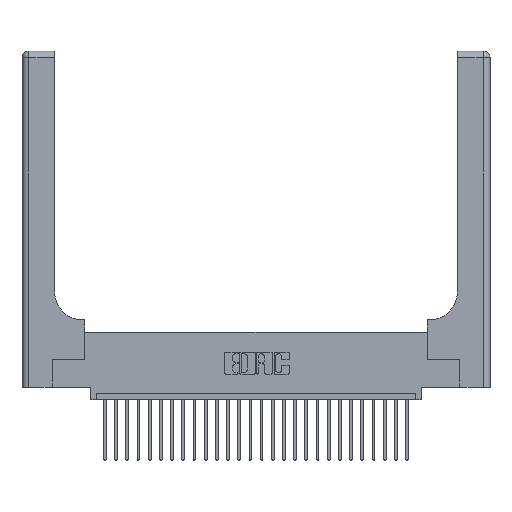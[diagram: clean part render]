
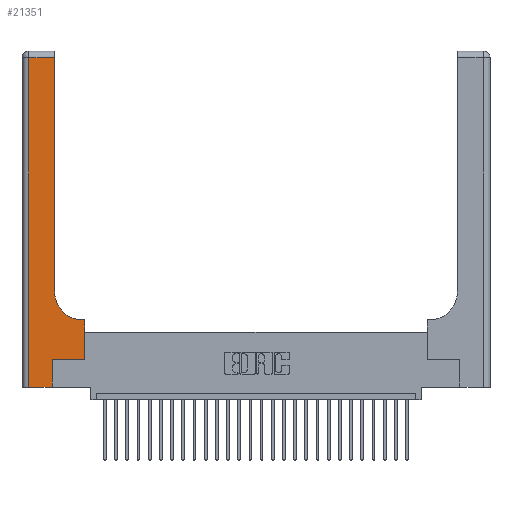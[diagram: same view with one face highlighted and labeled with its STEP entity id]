
A CAD part, top view. The second image highlights one B-rep face of the part: STEP entity #21351.
In plain terms, the highlighted planar face has unit normal (0, 0, 1).
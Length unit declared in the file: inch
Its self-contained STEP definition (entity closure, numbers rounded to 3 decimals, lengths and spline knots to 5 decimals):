
#375 = ORIENTED_EDGE ( 'NONE', *, *, #5644, .T. ) ;
#582 = CARTESIAN_POINT ( 'NONE',  ( 0.5585, 0.6, 0.37 ) ) ;
#1307 = VECTOR ( 'NONE', #10554, 39.37008 ) ;
#1419 = CARTESIAN_POINT ( 'NONE',  ( 0.2915, 0.6, 0.37 ) ) ;
#1467 = DIRECTION ( 'NONE',  ( 0., -1., 0. ) ) ;
#1536 = VERTEX_POINT ( 'NONE', #19108 ) ;
#2348 = CARTESIAN_POINT ( 'NONE',  ( 0.06, 0., 0.37 ) ) ;
#2480 = VERTEX_POINT ( 'NONE', #25996 ) ;
#2913 = EDGE_CURVE ( 'NONE', #25696, #2480, #7403, .T. ) ;
#3525 = DIRECTION ( 'NONE',  ( 0., 0., -1. ) ) ;
#3562 = DIRECTION ( 'NONE',  ( 1., 0., 0. ) ) ;
#3959 = CARTESIAN_POINT ( 'NONE',  ( 0.269, 0.25, 0.37 ) ) ;
#4008 = DIRECTION ( 'NONE',  ( 0., 1., 0. ) ) ;
#4486 = CARTESIAN_POINT ( 'NONE',  ( 0.5415, 0.85, 0.37 ) ) ;
#4943 = EDGE_CURVE ( 'NONE', #8313, #19720, #7279, .T. ) ;
#5218 = VECTOR ( 'NONE', #24473, 39.37008 ) ;
#5644 = EDGE_CURVE ( 'NONE', #8688, #8313, #22998, .T. ) ;
#5847 = DIRECTION ( 'NONE',  ( 1., 0., 0. ) ) ;
#5928 = CARTESIAN_POINT ( 'NONE',  ( 0.06, 3., 0.37 ) ) ;
#6504 = DIRECTION ( 'NONE',  ( 1., 0., 0. ) ) ;
#6826 = VECTOR ( 'NONE', #17107, 39.37008 ) ;
#7279 = LINE ( 'NONE', #9196, #5218 ) ;
#7403 = LINE ( 'NONE', #1419, #1307 ) ;
#7588 = VECTOR ( 'NONE', #3562, 39.37008 ) ;
#7600 = EDGE_CURVE ( 'NONE', #11409, #1536, #8986, .T. ) ;
#7817 = AXIS2_PLACEMENT_3D ( 'NONE', #14299, #3525, #7922 ) ;
#7922 = DIRECTION ( 'NONE',  ( -1., 0., 0. ) ) ;
#8313 = VERTEX_POINT ( 'NONE', #17157 ) ;
#8688 = VERTEX_POINT ( 'NONE', #23315 ) ;
#8885 = ORIENTED_EDGE ( 'NONE', *, *, #4943, .T. ) ;
#8986 = LINE ( 'NONE', #10336, #14761 ) ;
#9196 = CARTESIAN_POINT ( 'NONE',  ( 0., 2.94, 0.37 ) ) ;
#9477 = VERTEX_POINT ( 'NONE', #19957 ) ;
#10061 = ORIENTED_EDGE ( 'NONE', *, *, #15524, .T. ) ;
#10336 = CARTESIAN_POINT ( 'NONE',  ( 0.269, 0.25, 0.37 ) ) ;
#10338 = LINE ( 'NONE', #18715, #7588 ) ;
#10554 = DIRECTION ( 'NONE',  ( -1., 0., 0. ) ) ;
#10660 = EDGE_LOOP ( 'NONE', ( #375, #8885, #24581, #14808, #17787, #14865, #24493, #17031, #10061 ) ) ;
#11409 = VERTEX_POINT ( 'NONE', #3959 ) ;
#12402 = CARTESIAN_POINT ( 'NONE',  ( 0.2915, 3., 0.37 ) ) ;
#12955 = CIRCLE ( 'NONE', #24403, 0.25 ) ;
#14299 = CARTESIAN_POINT ( 'NONE',  ( 0., 3., 0.37 ) ) ;
#14342 = LINE ( 'NONE', #18221, #19476 ) ;
#14761 = VECTOR ( 'NONE', #5847, 39.37008 ) ;
#14808 = ORIENTED_EDGE ( 'NONE', *, *, #19629, .T. ) ;
#14865 = ORIENTED_EDGE ( 'NONE', *, *, #7600, .T. ) ;
#15524 = EDGE_CURVE ( 'NONE', #2480, #8688, #12955, .T. ) ;
#16726 = EDGE_CURVE ( 'NONE', #19720, #23976, #28287, .T. ) ;
#16909 = CARTESIAN_POINT ( 'NONE',  ( 0.06, 2.94, 0.37 ) ) ;
#17031 = ORIENTED_EDGE ( 'NONE', *, *, #2913, .T. ) ;
#17107 = DIRECTION ( 'NONE',  ( 0., 1., 0. ) ) ;
#17157 = CARTESIAN_POINT ( 'NONE',  ( 0.2915, 2.94, 0.37 ) ) ;
#17787 = ORIENTED_EDGE ( 'NONE', *, *, #23451, .T. ) ;
#18221 = CARTESIAN_POINT ( 'NONE',  ( 0.269, 0., 0.37 ) ) ;
#18327 = VECTOR ( 'NONE', #1467, 39.37008 ) ;
#18715 = CARTESIAN_POINT ( 'NONE',  ( 0., 0., 0.37 ) ) ;
#19108 = CARTESIAN_POINT ( 'NONE',  ( 0.5585, 0.25, 0.37 ) ) ;
#19476 = VECTOR ( 'NONE', #24892, 39.37008 ) ;
#19629 = EDGE_CURVE ( 'NONE', #23976, #9477, #10338, .T. ) ;
#19720 = VERTEX_POINT ( 'NONE', #16909 ) ;
#19957 = CARTESIAN_POINT ( 'NONE',  ( 0.269, 0., 0.37 ) ) ;
#20590 = FACE_OUTER_BOUND ( 'NONE', #10660, .T. ) ;
#21351 = ADVANCED_FACE ( 'NONE', ( #20590 ), #27404, .F. ) ;
#21433 = CARTESIAN_POINT ( 'NONE',  ( 0.5585, 0.25, 0.37 ) ) ;
#22178 = LINE ( 'NONE', #21433, #6826 ) ;
#22998 = LINE ( 'NONE', #12402, #27077 ) ;
#23315 = CARTESIAN_POINT ( 'NONE',  ( 0.2915, 0.85, 0.37 ) ) ;
#23451 = EDGE_CURVE ( 'NONE', #9477, #11409, #14342, .T. ) ;
#23872 = DIRECTION ( 'NONE',  ( 0., 0., -1. ) ) ;
#23976 = VERTEX_POINT ( 'NONE', #2348 ) ;
#24403 = AXIS2_PLACEMENT_3D ( 'NONE', #4486, #23872, #6504 ) ;
#24473 = DIRECTION ( 'NONE',  ( -1., 0., 0. ) ) ;
#24493 = ORIENTED_EDGE ( 'NONE', *, *, #26704, .T. ) ;
#24581 = ORIENTED_EDGE ( 'NONE', *, *, #16726, .T. ) ;
#24892 = DIRECTION ( 'NONE',  ( 0., 1., 0. ) ) ;
#25696 = VERTEX_POINT ( 'NONE', #582 ) ;
#25996 = CARTESIAN_POINT ( 'NONE',  ( 0.5415, 0.6, 0.37 ) ) ;
#26704 = EDGE_CURVE ( 'NONE', #1536, #25696, #22178, .T. ) ;
#27077 = VECTOR ( 'NONE', #4008, 39.37008 ) ;
#27404 = PLANE ( 'NONE',  #7817 ) ;
#28287 = LINE ( 'NONE', #5928, #18327 ) ;
